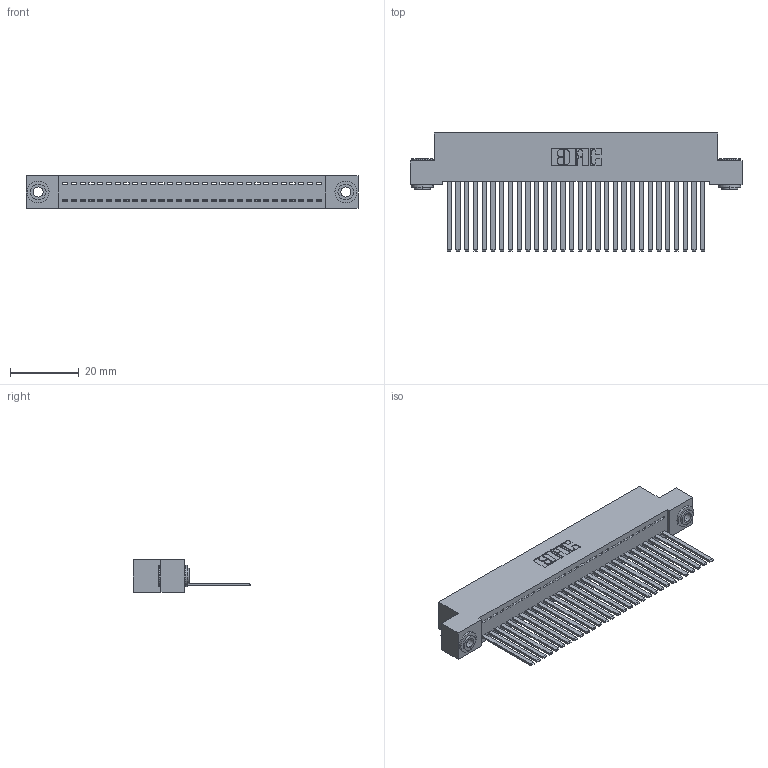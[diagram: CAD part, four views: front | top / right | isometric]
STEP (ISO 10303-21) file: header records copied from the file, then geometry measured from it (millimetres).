
FILE_DESCRIPTION (( 'STEP AP203' ), '1' );
FILE_NAME ('342-030-544-103.STEP', '2019-10-02T04:52:01', ( '' ), ( '' ), 'SwSTEP 2.0', 'SolidWorks 2016', '' );
FILE_SCHEMA (( 'CONFIG_CONTROL_DESIGN' ));
Length unit declared in the file: inch
Products named in the file (4): 342-030-544-103; 342 Part_.156 TH; 345-292-001_345-293-144; 342-250-002_345-250-002-102
Assembly tree (33 placements, depth 2):
  342-030-544-103
    342 Part_.156 TH
    345-292-001_345-293-144  x30
    342-250-002_345-250-002-102  x2
Bounding box: 96.52 x 34.3 x 9.4 mm (x, y, z)
Volume: 8788.9 mm3; surface area: 13897.1 mm2
Topology: 33 solids, 33 shells, 1708 faces, 5115 edges, 3366 vertices
Faces by surface type: plane 1216, cylinder 484, cone 8
Entity records: 20226 total; most frequent: CARTESIAN_POINT 3467, ORIENTED_EDGE 3426, DIRECTION 2979, EDGE_CURVE 1713, VECTOR 1565, LINE 1565, VERTEX_POINT 1138, AXIS2_PLACEMENT_3D 707
